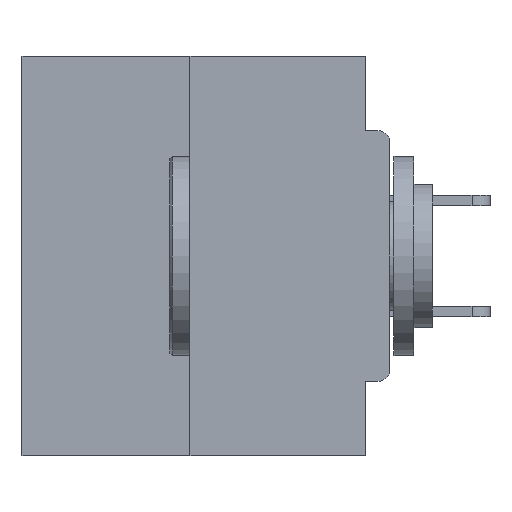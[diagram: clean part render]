
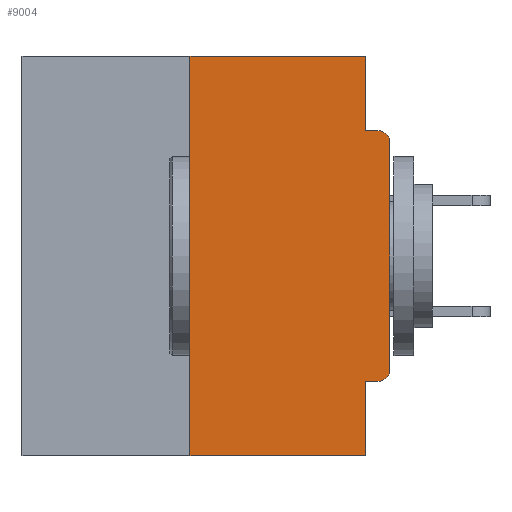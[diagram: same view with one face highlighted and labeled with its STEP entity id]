
A CAD part, left-side view. The second image highlights one B-rep face of the part: STEP entity #9004.
In plain terms, the highlighted planar face has unit normal (-1, 0, 0).
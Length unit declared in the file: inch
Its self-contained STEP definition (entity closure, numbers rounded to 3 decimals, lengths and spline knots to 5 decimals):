
#451 = PLANE ( 'NONE',  #1922 ) ;
#757 = VERTEX_POINT ( 'NONE', #4536 ) ;
#919 = VECTOR ( 'NONE', #21980, 39.37008 ) ;
#994 = LINE ( 'NONE', #19488, #21302 ) ;
#1095 = EDGE_CURVE ( 'NONE', #4886, #31557, #30598, .T. ) ;
#1410 = CARTESIAN_POINT ( 'NONE',  ( 0., 0.46, 0. ) ) ;
#1922 = AXIS2_PLACEMENT_3D ( 'NONE', #3217, #23040, #25479 ) ;
#2041 = LINE ( 'NONE', #24874, #17603 ) ;
#2106 = CARTESIAN_POINT ( 'NONE',  ( 0., 0.015, -0.1085 ) ) ;
#2372 = CARTESIAN_POINT ( 'NONE',  ( 0., 0.015, -0.4065 ) ) ;
#2642 = EDGE_CURVE ( 'NONE', #17270, #4886, #2041, .T. ) ;
#3217 = CARTESIAN_POINT ( 'NONE',  ( 0., 0.46, 0. ) ) ;
#3566 = EDGE_CURVE ( 'NONE', #32744, #21332, #16237, .T. ) ;
#3800 = CIRCLE ( 'NONE', #23018, 0.015 ) ;
#3911 = CARTESIAN_POINT ( 'NONE',  ( 0., 0.015, -0.0935 ) ) ;
#4026 = CARTESIAN_POINT ( 'NONE',  ( 0., 0.015, -0.3915 ) ) ;
#4536 = CARTESIAN_POINT ( 'NONE',  ( 0., 0.031, -0.4065 ) ) ;
#4886 = VERTEX_POINT ( 'NONE', #29508 ) ;
#5413 = CARTESIAN_POINT ( 'NONE',  ( 0., 0.25, -0.5 ) ) ;
#5899 = VECTOR ( 'NONE', #26533, 39.37008 ) ;
#5924 = VECTOR ( 'NONE', #6375, 39.37008 ) ;
#6193 = CARTESIAN_POINT ( 'NONE',  ( 0., 0.25, 0. ) ) ;
#6375 = DIRECTION ( 'NONE',  ( 0., -1., 0. ) ) ;
#6731 = DIRECTION ( 'NONE',  ( -1., 0., 0. ) ) ;
#6840 = ORIENTED_EDGE ( 'NONE', *, *, #2642, .T. ) ;
#7913 = CARTESIAN_POINT ( 'NONE',  ( 0., 0.031, -0.5 ) ) ;
#8384 = DIRECTION ( 'NONE',  ( 0., 0., 1. ) ) ;
#8427 = FACE_OUTER_BOUND ( 'NONE', #26319, .T. ) ;
#8824 = CARTESIAN_POINT ( 'NONE',  ( 0., 0., -0.0935 ) ) ;
#9004 = ADVANCED_FACE ( 'NONE', ( #8427 ), #451, .F. ) ;
#9145 = ORIENTED_EDGE ( 'NONE', *, *, #33941, .T. ) ;
#9154 = ORIENTED_EDGE ( 'NONE', *, *, #3566, .F. ) ;
#9440 = EDGE_CURVE ( 'NONE', #17952, #32744, #13573, .T. ) ;
#10612 = CARTESIAN_POINT ( 'NONE',  ( 0., 0.031, -0.0935 ) ) ;
#10817 = AXIS2_PLACEMENT_3D ( 'NONE', #2106, #26791, #29578 ) ;
#11572 = EDGE_CURVE ( 'NONE', #21332, #25995, #19389, .T. ) ;
#13573 = LINE ( 'NONE', #22986, #23505 ) ;
#14413 = VERTEX_POINT ( 'NONE', #27842 ) ;
#15471 = ORIENTED_EDGE ( 'NONE', *, *, #25388, .F. ) ;
#15908 = EDGE_CURVE ( 'NONE', #25995, #31557, #19264, .T. ) ;
#16237 = LINE ( 'NONE', #1410, #5899 ) ;
#16653 = ORIENTED_EDGE ( 'NONE', *, *, #31180, .T. ) ;
#17270 = VERTEX_POINT ( 'NONE', #28387 ) ;
#17603 = VECTOR ( 'NONE', #8384, 39.37008 ) ;
#17952 = VERTEX_POINT ( 'NONE', #5413 ) ;
#19264 = LINE ( 'NONE', #8824, #5924 ) ;
#19389 = LINE ( 'NONE', #30165, #21586 ) ;
#19429 = ORIENTED_EDGE ( 'NONE', *, *, #9440, .F. ) ;
#19488 = CARTESIAN_POINT ( 'NONE',  ( 0., 0.46, -0.5 ) ) ;
#19823 = EDGE_CURVE ( 'NONE', #757, #14413, #27301, .T. ) ;
#20326 = DIRECTION ( 'NONE',  ( 0., 0., -1. ) ) ;
#20968 = ORIENTED_EDGE ( 'NONE', *, *, #15908, .F. ) ;
#21302 = VECTOR ( 'NONE', #25179, 39.37008 ) ;
#21332 = VERTEX_POINT ( 'NONE', #35146 ) ;
#21586 = VECTOR ( 'NONE', #32573, 39.37008 ) ;
#21980 = DIRECTION ( 'NONE',  ( 0., 0., -1. ) ) ;
#22986 = CARTESIAN_POINT ( 'NONE',  ( 0., 0.25, 0. ) ) ;
#23018 = AXIS2_PLACEMENT_3D ( 'NONE', #4026, #6731, #20326 ) ;
#23040 = DIRECTION ( 'NONE',  ( 1., 0., 0. ) ) ;
#23505 = VECTOR ( 'NONE', #34223, 39.37008 ) ;
#24874 = CARTESIAN_POINT ( 'NONE',  ( 0., 0., 0. ) ) ;
#25179 = DIRECTION ( 'NONE',  ( 0., -1., 0. ) ) ;
#25388 = EDGE_CURVE ( 'NONE', #28112, #757, #28188, .T. ) ;
#25479 = DIRECTION ( 'NONE',  ( 0., 0., -1. ) ) ;
#25606 = ORIENTED_EDGE ( 'NONE', *, *, #11572, .F. ) ;
#25995 = VERTEX_POINT ( 'NONE', #10612 ) ;
#26319 = EDGE_LOOP ( 'NONE', ( #9154, #19429, #16653, #31167, #15471, #9145, #6840, #34843, #20968, #25606 ) ) ;
#26533 = DIRECTION ( 'NONE',  ( 0., -1., 0. ) ) ;
#26791 = DIRECTION ( 'NONE',  ( -1., 0., 0. ) ) ;
#27301 = LINE ( 'NONE', #7913, #919 ) ;
#27842 = CARTESIAN_POINT ( 'NONE',  ( 0., 0.031, -0.5 ) ) ;
#28112 = VERTEX_POINT ( 'NONE', #2372 ) ;
#28188 = LINE ( 'NONE', #29210, #34613 ) ;
#28387 = CARTESIAN_POINT ( 'NONE',  ( 0., 0., -0.3915 ) ) ;
#29210 = CARTESIAN_POINT ( 'NONE',  ( 0., 0., -0.4065 ) ) ;
#29508 = CARTESIAN_POINT ( 'NONE',  ( 0., 0., -0.1085 ) ) ;
#29578 = DIRECTION ( 'NONE',  ( 0., 0., -1. ) ) ;
#30165 = CARTESIAN_POINT ( 'NONE',  ( 0., 0.031, 0. ) ) ;
#30598 = CIRCLE ( 'NONE', #10817, 0.015 ) ;
#31167 = ORIENTED_EDGE ( 'NONE', *, *, #19823, .F. ) ;
#31180 = EDGE_CURVE ( 'NONE', #17952, #14413, #994, .T. ) ;
#31557 = VERTEX_POINT ( 'NONE', #3911 ) ;
#32044 = DIRECTION ( 'NONE',  ( 0., 1., 0. ) ) ;
#32573 = DIRECTION ( 'NONE',  ( 0., 0., -1. ) ) ;
#32744 = VERTEX_POINT ( 'NONE', #6193 ) ;
#33941 = EDGE_CURVE ( 'NONE', #28112, #17270, #3800, .T. ) ;
#34223 = DIRECTION ( 'NONE',  ( 0., 0., 1. ) ) ;
#34613 = VECTOR ( 'NONE', #32044, 39.37008 ) ;
#34843 = ORIENTED_EDGE ( 'NONE', *, *, #1095, .T. ) ;
#35146 = CARTESIAN_POINT ( 'NONE',  ( 0., 0.031, 0. ) ) ;
